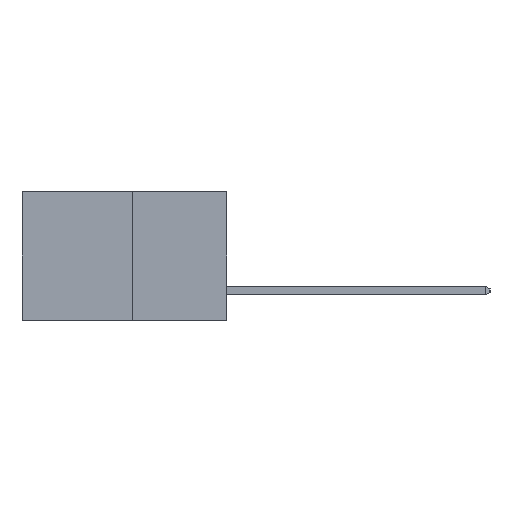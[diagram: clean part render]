
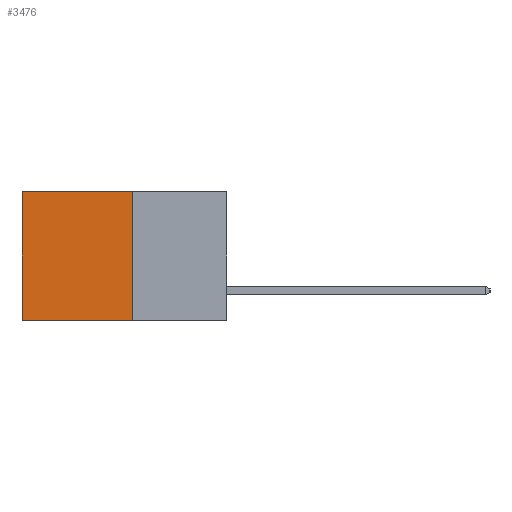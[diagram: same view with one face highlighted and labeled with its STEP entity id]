
A CAD part, left-side view. The second image highlights one B-rep face of the part: STEP entity #3476.
In plain terms, the highlighted planar face has unit normal (-1, 0, 0).
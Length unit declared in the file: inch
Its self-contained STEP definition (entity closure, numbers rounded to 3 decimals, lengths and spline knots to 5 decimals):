
#109 = ORIENTED_EDGE ( 'NONE', *, *, #7251, .T. ) ;
#299 = DIRECTION ( 'NONE',  ( 0., 1., 0. ) ) ;
#328 = LINE ( 'NONE', #1193, #4303 ) ;
#688 = PLANE ( 'NONE',  #3915 ) ;
#836 = FACE_OUTER_BOUND ( 'NONE', #4637, .T. ) ;
#979 = CARTESIAN_POINT ( 'NONE',  ( 0.277, 0.27, 0. ) ) ;
#1156 = CARTESIAN_POINT ( 'NONE',  ( 0.277, 0.59, -0.37 ) ) ;
#1193 = CARTESIAN_POINT ( 'NONE',  ( 0.277, 0.27, -0.37 ) ) ;
#1763 = ORIENTED_EDGE ( 'NONE', *, *, #7012, .F. ) ;
#2031 = CARTESIAN_POINT ( 'NONE',  ( 0.277, 0.27, 0. ) ) ;
#2106 = LINE ( 'NONE', #2031, #9598 ) ;
#3162 = VERTEX_POINT ( 'NONE', #979 ) ;
#3306 = DIRECTION ( 'NONE',  ( 0., 0., -1. ) ) ;
#3476 = ADVANCED_FACE ( 'NONE', ( #836 ), #688, .F. ) ;
#3915 = AXIS2_PLACEMENT_3D ( 'NONE', #5771, #9203, #6212 ) ;
#4303 = VECTOR ( 'NONE', #299, 39.37008 ) ;
#4321 = CARTESIAN_POINT ( 'NONE',  ( 0.277, 0.59, -0.37 ) ) ;
#4453 = VECTOR ( 'NONE', #3306, 39.37008 ) ;
#4622 = EDGE_CURVE ( 'NONE', #3162, #9485, #2106, .T. ) ;
#4637 = EDGE_LOOP ( 'NONE', ( #109, #6087, #1763, #9666 ) ) ;
#5452 = CARTESIAN_POINT ( 'NONE',  ( 0.277, 0.27, -0.37 ) ) ;
#5771 = CARTESIAN_POINT ( 'NONE',  ( 0.277, 0.27, -0.37 ) ) ;
#5941 = CARTESIAN_POINT ( 'NONE',  ( 0.277, 0.59, 0. ) ) ;
#6065 = VERTEX_POINT ( 'NONE', #5452 ) ;
#6087 = ORIENTED_EDGE ( 'NONE', *, *, #8645, .F. ) ;
#6212 = DIRECTION ( 'NONE',  ( 0., 0., -1. ) ) ;
#6768 = VECTOR ( 'NONE', #6777, 39.37008 ) ;
#6777 = DIRECTION ( 'NONE',  ( 0., 0., -1. ) ) ;
#6986 = CARTESIAN_POINT ( 'NONE',  ( 0.277, 0.27, -0.37 ) ) ;
#7012 = EDGE_CURVE ( 'NONE', #3162, #6065, #8777, .T. ) ;
#7251 = EDGE_CURVE ( 'NONE', #9485, #8837, #8221, .T. ) ;
#8221 = LINE ( 'NONE', #4321, #4453 ) ;
#8281 = DIRECTION ( 'NONE',  ( 0., 1., 0. ) ) ;
#8645 = EDGE_CURVE ( 'NONE', #6065, #8837, #328, .T. ) ;
#8777 = LINE ( 'NONE', #6986, #6768 ) ;
#8837 = VERTEX_POINT ( 'NONE', #1156 ) ;
#9203 = DIRECTION ( 'NONE',  ( 1., 0., 0. ) ) ;
#9485 = VERTEX_POINT ( 'NONE', #5941 ) ;
#9598 = VECTOR ( 'NONE', #8281, 39.37008 ) ;
#9666 = ORIENTED_EDGE ( 'NONE', *, *, #4622, .T. ) ;
